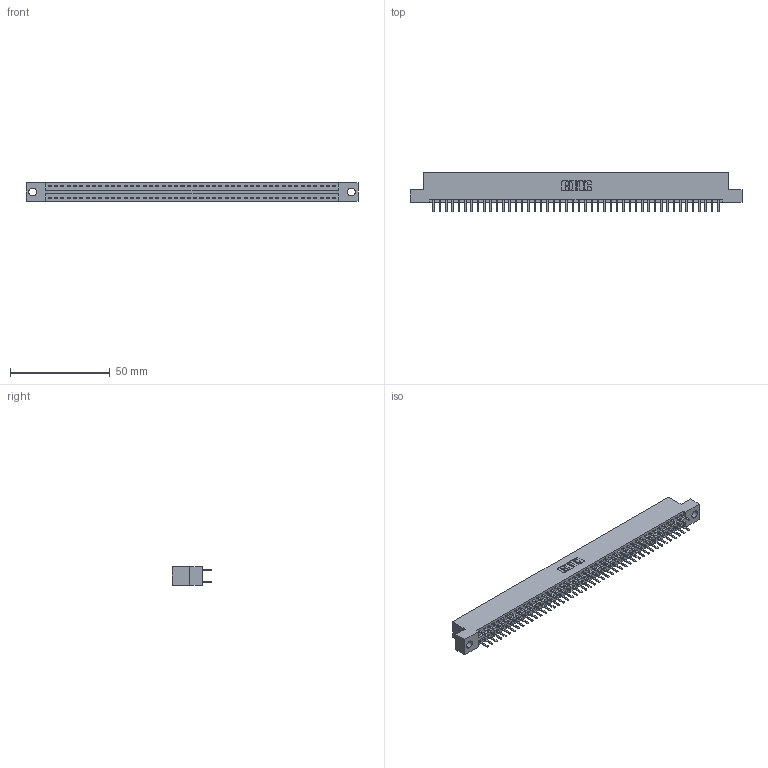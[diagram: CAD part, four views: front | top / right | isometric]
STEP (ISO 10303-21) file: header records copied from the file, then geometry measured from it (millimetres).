
FILE_DESCRIPTION (( 'STEP AP203' ), '1' );
FILE_NAME ('396-092-520-204.STEP', '2019-10-31T02:21:23', ( '' ), ( '' ), 'SwSTEP 2.0', 'SolidWorks 2016', '' );
FILE_SCHEMA (( 'CONFIG_CONTROL_DESIGN' ));
Length unit declared in the file: inch
Products named in the file (3): 345-292-001_345-293-120; 396-092-520-204; 346 Part_Flush Mounting Lugs - 0.156 Dia-TH
Assembly tree (93 placements, depth 2):
  396-092-520-204
    346 Part_Flush Mounting Lugs - 0.156 Dia-TH
    345-292-001_345-293-120  x92
Bounding box: 166.62 x 20.02 x 9.4 mm (x, y, z)
Volume: 16150.7 mm3; surface area: 21981.6 mm2
Topology: 93 solids, 93 shells, 5274 faces, 15325 edges, 9970 vertices
Faces by surface type: plane 3480, cylinder 1794
Entity records: 29599 total; most frequent: CARTESIAN_POINT 4884, ORIENTED_EDGE 4806, DIRECTION 4343, EDGE_CURVE 2403, VECTOR 2083, LINE 2083, VERTEX_POINT 1598, AXIS2_PLACEMENT_3D 1130
